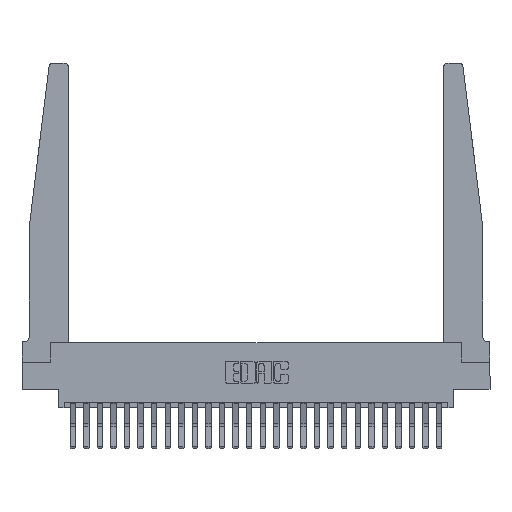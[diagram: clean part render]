
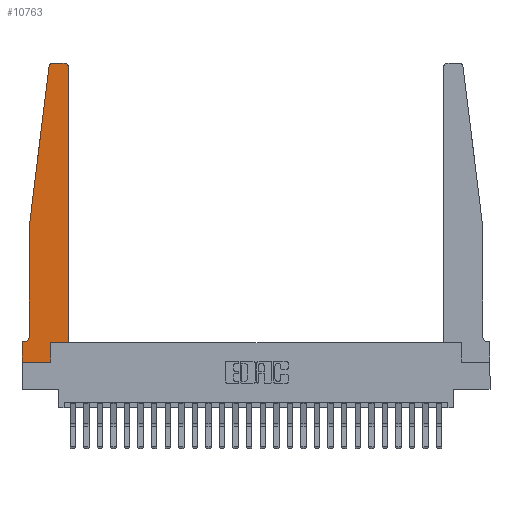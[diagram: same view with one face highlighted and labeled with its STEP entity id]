
A CAD part, top view. The second image highlights one B-rep face of the part: STEP entity #10763.
In plain terms, the highlighted planar face has unit normal (0, 0, 1).
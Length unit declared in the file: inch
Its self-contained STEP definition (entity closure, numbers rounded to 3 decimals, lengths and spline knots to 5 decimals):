
#319 = DIRECTION ( 'NONE',  ( 1., 0., 0. ) ) ;
#411 = LINE ( 'NONE', #24429, #19869 ) ;
#954 = CIRCLE ( 'NONE', #3928, 0.03 ) ;
#1139 = DIRECTION ( 'NONE',  ( -0.122, -0.992, 0. ) ) ;
#1254 = EDGE_CURVE ( 'NONE', #6209, #11422, #954, .T. ) ;
#1485 = CARTESIAN_POINT ( 'NONE',  ( 0.065, 0.2375, 0.37 ) ) ;
#2180 = VERTEX_POINT ( 'NONE', #4039 ) ;
#2221 = EDGE_LOOP ( 'NONE', ( #15629, #5145, #14897, #17383, #10460, #9044, #7195, #16601, #16907, #2382, #12165, #12483 ) ) ;
#2382 = ORIENTED_EDGE ( 'NONE', *, *, #12498, .T. ) ;
#2388 = LINE ( 'NONE', #22470, #8195 ) ;
#3026 = AXIS2_PLACEMENT_3D ( 'NONE', #23598, #12007, #319 ) ;
#3216 = EDGE_CURVE ( 'NONE', #11422, #13267, #7464, .T. ) ;
#3396 = VERTEX_POINT ( 'NONE', #3988 ) ;
#3750 = EDGE_CURVE ( 'NONE', #2180, #3396, #411, .T. ) ;
#3873 = DIRECTION ( 'NONE',  ( 0., 0., -1. ) ) ;
#3928 = AXIS2_PLACEMENT_3D ( 'NONE', #5234, #18799, #7203 ) ;
#3988 = CARTESIAN_POINT ( 'NONE',  ( 0.065, 1.25, 0.37 ) ) ;
#3997 = EDGE_CURVE ( 'NONE', #21986, #15900, #24711, .T. ) ;
#4039 = CARTESIAN_POINT ( 'NONE',  ( 0.24675, 2.72367, 0.37 ) ) ;
#4228 = DIRECTION ( 'NONE',  ( 0., 0., 1. ) ) ;
#4275 = CARTESIAN_POINT ( 'NONE',  ( 0.27653, 2.75, 0.37 ) ) ;
#5145 = ORIENTED_EDGE ( 'NONE', *, *, #11891, .T. ) ;
#5234 = CARTESIAN_POINT ( 'NONE',  ( 0.395, 2.72, 0.37 ) ) ;
#5453 = CARTESIAN_POINT ( 'NONE',  ( 0.25, 2.75, 0.37 ) ) ;
#5857 = DIRECTION ( 'NONE',  ( 0., 1., 0. ) ) ;
#5882 = VERTEX_POINT ( 'NONE', #11806 ) ;
#5921 = EDGE_CURVE ( 'NONE', #18439, #6209, #7658, .T. ) ;
#6209 = VERTEX_POINT ( 'NONE', #7351 ) ;
#6478 = AXIS2_PLACEMENT_3D ( 'NONE', #15523, #3873, #17482 ) ;
#6661 = CARTESIAN_POINT ( 'NONE',  ( 0., 0., 0.37 ) ) ;
#7195 = ORIENTED_EDGE ( 'NONE', *, *, #9637, .T. ) ;
#7203 = DIRECTION ( 'NONE',  ( 1., 0., 0. ) ) ;
#7306 = LINE ( 'NONE', #6661, #16390 ) ;
#7351 = CARTESIAN_POINT ( 'NONE',  ( 0.425, 2.72, 0.37 ) ) ;
#7405 = DIRECTION ( 'NONE',  ( -1., 0., 0. ) ) ;
#7464 = LINE ( 'NONE', #5453, #13243 ) ;
#7658 = LINE ( 'NONE', #19680, #17376 ) ;
#7713 = CARTESIAN_POINT ( 'NONE',  ( 0.065, 0.1875, 0.37 ) ) ;
#8070 = DIRECTION ( 'NONE',  ( 0., 1., 0. ) ) ;
#8117 = DIRECTION ( 'NONE',  ( 1., 0., 0. ) ) ;
#8195 = VECTOR ( 'NONE', #10903, 39.37008 ) ;
#8382 = CARTESIAN_POINT ( 'NONE',  ( 0.395, 2.75, 0.37 ) ) ;
#8536 = DIRECTION ( 'NONE',  ( 0., -1., 0. ) ) ;
#8621 = CARTESIAN_POINT ( 'NONE',  ( 0., 0.1875, 0.37 ) ) ;
#8659 = EDGE_CURVE ( 'NONE', #16923, #5882, #17671, .T. ) ;
#8773 = FACE_OUTER_BOUND ( 'NONE', #2221, .T. ) ;
#9044 = ORIENTED_EDGE ( 'NONE', *, *, #3997, .T. ) ;
#9637 = EDGE_CURVE ( 'NONE', #15900, #21965, #7306, .T. ) ;
#9797 = CARTESIAN_POINT ( 'NONE',  ( 0.2605, 0.18, 0.37 ) ) ;
#9960 = CARTESIAN_POINT ( 'NONE',  ( 0.425, 0.18, 0.37 ) ) ;
#10333 = EDGE_CURVE ( 'NONE', #3396, #22400, #2388, .T. ) ;
#10460 = ORIENTED_EDGE ( 'NONE', *, *, #12406, .T. ) ;
#10763 = ADVANCED_FACE ( 'NONE', ( #8773 ), #15864, .T. ) ;
#10903 = DIRECTION ( 'NONE',  ( 0., -1., 0. ) ) ;
#11422 = VERTEX_POINT ( 'NONE', #8382 ) ;
#11806 = CARTESIAN_POINT ( 'NONE',  ( 0.2605, 0.18, 0.37 ) ) ;
#11891 = EDGE_CURVE ( 'NONE', #13267, #2180, #16004, .T. ) ;
#12007 = DIRECTION ( 'NONE',  ( 0., 0., 1. ) ) ;
#12165 = ORIENTED_EDGE ( 'NONE', *, *, #5921, .T. ) ;
#12363 = CARTESIAN_POINT ( 'NONE',  ( 0.2605, 0., 0.37 ) ) ;
#12406 = EDGE_CURVE ( 'NONE', #22400, #21986, #19299, .T. ) ;
#12483 = ORIENTED_EDGE ( 'NONE', *, *, #1254, .T. ) ;
#12498 = EDGE_CURVE ( 'NONE', #5882, #18439, #18077, .T. ) ;
#12605 = VECTOR ( 'NONE', #8117, 39.37008 ) ;
#13231 = EDGE_CURVE ( 'NONE', #21965, #16923, #22280, .T. ) ;
#13243 = VECTOR ( 'NONE', #7405, 39.37008 ) ;
#13267 = VERTEX_POINT ( 'NONE', #4275 ) ;
#13395 = CARTESIAN_POINT ( 'NONE',  ( 0.425, 0.18, 0.37 ) ) ;
#14163 = VECTOR ( 'NONE', #21503, 39.37008 ) ;
#14897 = ORIENTED_EDGE ( 'NONE', *, *, #3750, .T. ) ;
#15523 = CARTESIAN_POINT ( 'NONE',  ( 0.015, 0.2375, 0.37 ) ) ;
#15629 = ORIENTED_EDGE ( 'NONE', *, *, #3216, .T. ) ;
#15864 = PLANE ( 'NONE',  #23890 ) ;
#15900 = VERTEX_POINT ( 'NONE', #8621 ) ;
#16004 = CIRCLE ( 'NONE', #3026, 0.03 ) ;
#16390 = VECTOR ( 'NONE', #8536, 39.37008 ) ;
#16601 = ORIENTED_EDGE ( 'NONE', *, *, #13231, .T. ) ;
#16907 = ORIENTED_EDGE ( 'NONE', *, *, #8659, .T. ) ;
#16923 = VERTEX_POINT ( 'NONE', #12363 ) ;
#17376 = VECTOR ( 'NONE', #8070, 39.37008 ) ;
#17383 = ORIENTED_EDGE ( 'NONE', *, *, #10333, .T. ) ;
#17482 = DIRECTION ( 'NONE',  ( -1., 0., 0. ) ) ;
#17671 = LINE ( 'NONE', #9797, #22473 ) ;
#17804 = DIRECTION ( 'NONE',  ( 1., 0., 0. ) ) ;
#18077 = LINE ( 'NONE', #9960, #14163 ) ;
#18439 = VERTEX_POINT ( 'NONE', #13395 ) ;
#18799 = DIRECTION ( 'NONE',  ( 0., 0., 1. ) ) ;
#19299 = CIRCLE ( 'NONE', #6478, 0.05 ) ;
#19557 = VECTOR ( 'NONE', #23215, 39.37008 ) ;
#19680 = CARTESIAN_POINT ( 'NONE',  ( 0.425, 0.18, 0.37 ) ) ;
#19729 = CARTESIAN_POINT ( 'NONE',  ( 0., 0., 0.37 ) ) ;
#19869 = VECTOR ( 'NONE', #1139, 39.37008 ) ;
#21503 = DIRECTION ( 'NONE',  ( 1., 0., 0. ) ) ;
#21594 = CARTESIAN_POINT ( 'NONE',  ( 0., 0.1875, 0.37 ) ) ;
#21773 = CARTESIAN_POINT ( 'NONE',  ( 0., 0., 0.37 ) ) ;
#21965 = VERTEX_POINT ( 'NONE', #21773 ) ;
#21986 = VERTEX_POINT ( 'NONE', #23838 ) ;
#22280 = LINE ( 'NONE', #19729, #12605 ) ;
#22400 = VERTEX_POINT ( 'NONE', #1485 ) ;
#22470 = CARTESIAN_POINT ( 'NONE',  ( 0.065, 1.25, 0.37 ) ) ;
#22473 = VECTOR ( 'NONE', #5857, 39.37008 ) ;
#23215 = DIRECTION ( 'NONE',  ( -1., 0., 0. ) ) ;
#23598 = CARTESIAN_POINT ( 'NONE',  ( 0.27653, 2.72, 0.37 ) ) ;
#23838 = CARTESIAN_POINT ( 'NONE',  ( 0.015, 0.1875, 0.37 ) ) ;
#23890 = AXIS2_PLACEMENT_3D ( 'NONE', #21594, #4228, #17804 ) ;
#24429 = CARTESIAN_POINT ( 'NONE',  ( 0.065, 1.25, 0.37 ) ) ;
#24711 = LINE ( 'NONE', #7713, #19557 ) ;
